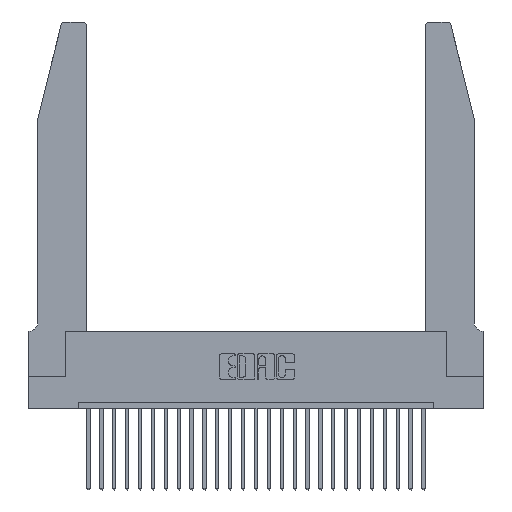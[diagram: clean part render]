
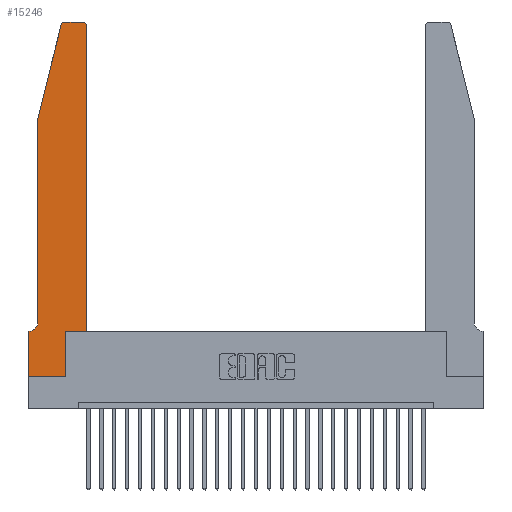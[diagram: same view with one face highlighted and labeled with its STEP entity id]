
A CAD part, top view. The second image highlights one B-rep face of the part: STEP entity #15246.
In plain terms, the highlighted planar face has unit normal (0, 0, 1).
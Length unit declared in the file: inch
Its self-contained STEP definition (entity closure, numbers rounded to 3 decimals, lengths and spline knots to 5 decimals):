
#135 = ORIENTED_EDGE ( 'NONE', *, *, #16452, .T. ) ;
#557 = VERTEX_POINT ( 'NONE', #26064 ) ;
#1004 = AXIS2_PLACEMENT_3D ( 'NONE', #1490, #18290, #1398 ) ;
#1007 = DIRECTION ( 'NONE',  ( 0., -1., 0. ) ) ;
#1112 = CARTESIAN_POINT ( 'NONE',  ( 0.0755, 2., 0.37 ) ) ;
#1114 = VERTEX_POINT ( 'NONE', #7480 ) ;
#1211 = DIRECTION ( 'NONE',  ( 0., 0., 1. ) ) ;
#1398 = DIRECTION ( 'NONE',  ( 1., 0., 0. ) ) ;
#1490 = CARTESIAN_POINT ( 'NONE',  ( 0.284, 2.72, 0.37 ) ) ;
#2289 = EDGE_CURVE ( 'NONE', #13863, #22838, #26358, .T. ) ;
#2352 = VECTOR ( 'NONE', #7096, 39.37008 ) ;
#2856 = CARTESIAN_POINT ( 'NONE',  ( 0.0755, 0.42, 0.37 ) ) ;
#2878 = CARTESIAN_POINT ( 'NONE',  ( 0.2865, 0.35, 0.37 ) ) ;
#2986 = VECTOR ( 'NONE', #24689, 39.37008 ) ;
#3426 = EDGE_CURVE ( 'NONE', #14115, #1114, #5640, .T. ) ;
#3467 = LINE ( 'NONE', #8801, #21521 ) ;
#3740 = CARTESIAN_POINT ( 'NONE',  ( 0.284, 2.75, 0.37 ) ) ;
#4015 = LINE ( 'NONE', #1112, #26580 ) ;
#4114 = CARTESIAN_POINT ( 'NONE',  ( 0.4505, 0.35, 0.37 ) ) ;
#5640 = CIRCLE ( 'NONE', #6545, 0.07 ) ;
#5718 = CARTESIAN_POINT ( 'NONE',  ( 0.2865, 0.35, 0.37 ) ) ;
#5940 = ORIENTED_EDGE ( 'NONE', *, *, #16201, .T. ) ;
#5990 = VERTEX_POINT ( 'NONE', #3740 ) ;
#6000 = DIRECTION ( 'NONE',  ( 0., 1., 0. ) ) ;
#6066 = ORIENTED_EDGE ( 'NONE', *, *, #16531, .T. ) ;
#6413 = CARTESIAN_POINT ( 'NONE',  ( 0.4205, 2.72, 0.37 ) ) ;
#6545 = AXIS2_PLACEMENT_3D ( 'NONE', #23772, #8843, #17477 ) ;
#6684 = DIRECTION ( 'NONE',  ( 1., 0., 0. ) ) ;
#6901 = EDGE_LOOP ( 'NONE', ( #21203, #26870, #24633, #14409, #8132, #12255, #135, #5940, #6066, #15319, #10232, #19906 ) ) ;
#7096 = DIRECTION ( 'NONE',  ( 1., 0., 0. ) ) ;
#7367 = AXIS2_PLACEMENT_3D ( 'NONE', #22468, #1211, #9940 ) ;
#7480 = CARTESIAN_POINT ( 'NONE',  ( 0.0055, 0.35, 0.37 ) ) ;
#7492 = CIRCLE ( 'NONE', #1004, 0.03 ) ;
#8132 = ORIENTED_EDGE ( 'NONE', *, *, #3426, .T. ) ;
#8532 = CARTESIAN_POINT ( 'NONE',  ( 0.4505, 0.35, 0.37 ) ) ;
#8604 = LINE ( 'NONE', #12268, #2986 ) ;
#8801 = CARTESIAN_POINT ( 'NONE',  ( 0.0755, 2., 0.37 ) ) ;
#8843 = DIRECTION ( 'NONE',  ( 0., 0., -1. ) ) ;
#9027 = VECTOR ( 'NONE', #6000, 39.37008 ) ;
#9142 = EDGE_CURVE ( 'NONE', #14101, #14115, #4015, .T. ) ;
#9940 = DIRECTION ( 'NONE',  ( 1., 0., 0. ) ) ;
#9967 = CARTESIAN_POINT ( 'NONE',  ( 0.4205, 2.75, 0.37 ) ) ;
#10232 = ORIENTED_EDGE ( 'NONE', *, *, #2289, .T. ) ;
#10242 = DIRECTION ( 'NONE',  ( 0., -1., 0. ) ) ;
#10446 = VECTOR ( 'NONE', #19627, 39.37008 ) ;
#10904 = DIRECTION ( 'NONE',  ( -1., 0., 0. ) ) ;
#11013 = DIRECTION ( 'NONE',  ( -0.239, -0.971, 0. ) ) ;
#11171 = CARTESIAN_POINT ( 'NONE',  ( 0., 0., 0.37 ) ) ;
#12178 = EDGE_CURVE ( 'NONE', #22838, #12629, #20593, .T. ) ;
#12255 = ORIENTED_EDGE ( 'NONE', *, *, #16478, .T. ) ;
#12268 = CARTESIAN_POINT ( 'NONE',  ( 0.0755, 0.35, 0.37 ) ) ;
#12629 = VERTEX_POINT ( 'NONE', #9967 ) ;
#12653 = CARTESIAN_POINT ( 'NONE',  ( 0.4505, 2.72, 0.37 ) ) ;
#13857 = VERTEX_POINT ( 'NONE', #23808 ) ;
#13863 = VERTEX_POINT ( 'NONE', #23637 ) ;
#14040 = VERTEX_POINT ( 'NONE', #21410 ) ;
#14101 = VERTEX_POINT ( 'NONE', #21386 ) ;
#14115 = VERTEX_POINT ( 'NONE', #2856 ) ;
#14409 = ORIENTED_EDGE ( 'NONE', *, *, #9142, .T. ) ;
#14882 = FACE_OUTER_BOUND ( 'NONE', #6901, .T. ) ;
#15042 = VERTEX_POINT ( 'NONE', #2878 ) ;
#15059 = VERTEX_POINT ( 'NONE', #21921 ) ;
#15069 = VECTOR ( 'NONE', #10904, 39.37008 ) ;
#15246 = ADVANCED_FACE ( 'NONE', ( #14882 ), #16074, .T. ) ;
#15319 = ORIENTED_EDGE ( 'NONE', *, *, #19020, .T. ) ;
#15875 = AXIS2_PLACEMENT_3D ( 'NONE', #6413, #25469, #6684 ) ;
#16074 = PLANE ( 'NONE',  #7367 ) ;
#16196 = CARTESIAN_POINT ( 'NONE',  ( 0., 0., 0.37 ) ) ;
#16201 = EDGE_CURVE ( 'NONE', #14040, #13857, #19762, .T. ) ;
#16376 = LINE ( 'NONE', #23373, #15069 ) ;
#16452 = EDGE_CURVE ( 'NONE', #15059, #14040, #23967, .T. ) ;
#16478 = EDGE_CURVE ( 'NONE', #1114, #15059, #8604, .T. ) ;
#16531 = EDGE_CURVE ( 'NONE', #13857, #15042, #26553, .T. ) ;
#17477 = DIRECTION ( 'NONE',  ( -1., 0., 0. ) ) ;
#18290 = DIRECTION ( 'NONE',  ( 0., 0., 1. ) ) ;
#19020 = EDGE_CURVE ( 'NONE', #15042, #13863, #25155, .T. ) ;
#19627 = DIRECTION ( 'NONE',  ( 1., 0., 0. ) ) ;
#19762 = LINE ( 'NONE', #11171, #2352 ) ;
#19906 = ORIENTED_EDGE ( 'NONE', *, *, #12178, .T. ) ;
#20409 = VECTOR ( 'NONE', #10242, 39.37008 ) ;
#20593 = CIRCLE ( 'NONE', #15875, 0.03 ) ;
#21203 = ORIENTED_EDGE ( 'NONE', *, *, #26381, .T. ) ;
#21386 = CARTESIAN_POINT ( 'NONE',  ( 0.0755, 2., 0.37 ) ) ;
#21410 = CARTESIAN_POINT ( 'NONE',  ( 0., 0., 0.37 ) ) ;
#21521 = VECTOR ( 'NONE', #11013, 39.37008 ) ;
#21921 = CARTESIAN_POINT ( 'NONE',  ( 0., 0.35, 0.37 ) ) ;
#21956 = EDGE_CURVE ( 'NONE', #5990, #557, #7492, .T. ) ;
#22468 = CARTESIAN_POINT ( 'NONE',  ( 0., 0.35, 0.37 ) ) ;
#22838 = VERTEX_POINT ( 'NONE', #12653 ) ;
#23373 = CARTESIAN_POINT ( 'NONE',  ( 0.2605, 2.75, 0.37 ) ) ;
#23637 = CARTESIAN_POINT ( 'NONE',  ( 0.4505, 0.35, 0.37 ) ) ;
#23772 = CARTESIAN_POINT ( 'NONE',  ( 0.0055, 0.42, 0.37 ) ) ;
#23808 = CARTESIAN_POINT ( 'NONE',  ( 0.2865, 0., 0.37 ) ) ;
#23849 = EDGE_CURVE ( 'NONE', #557, #14101, #3467, .T. ) ;
#23967 = LINE ( 'NONE', #16196, #20409 ) ;
#24589 = DIRECTION ( 'NONE',  ( 0., 1., 0. ) ) ;
#24633 = ORIENTED_EDGE ( 'NONE', *, *, #23849, .T. ) ;
#24689 = DIRECTION ( 'NONE',  ( -1., 0., 0. ) ) ;
#25155 = LINE ( 'NONE', #8532, #10446 ) ;
#25270 = VECTOR ( 'NONE', #24589, 39.37008 ) ;
#25469 = DIRECTION ( 'NONE',  ( 0., 0., 1. ) ) ;
#26064 = CARTESIAN_POINT ( 'NONE',  ( 0.25487, 2.72718, 0.37 ) ) ;
#26358 = LINE ( 'NONE', #4114, #9027 ) ;
#26381 = EDGE_CURVE ( 'NONE', #12629, #5990, #16376, .T. ) ;
#26553 = LINE ( 'NONE', #5718, #25270 ) ;
#26580 = VECTOR ( 'NONE', #1007, 39.37008 ) ;
#26870 = ORIENTED_EDGE ( 'NONE', *, *, #21956, .T. ) ;
